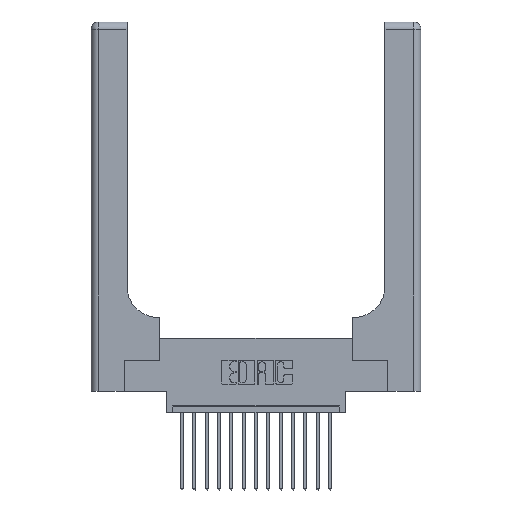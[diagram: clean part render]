
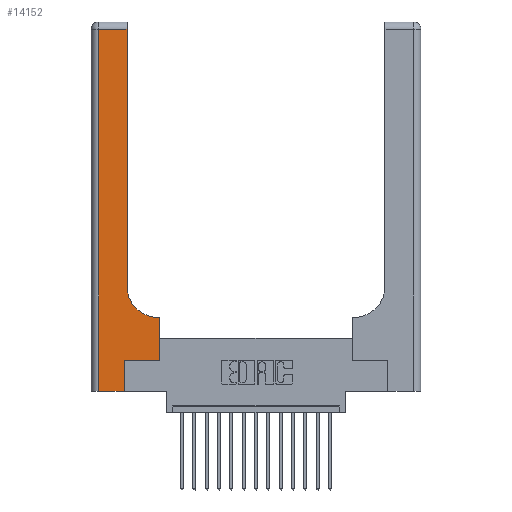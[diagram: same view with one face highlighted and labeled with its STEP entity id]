
A CAD part, top view. The second image highlights one B-rep face of the part: STEP entity #14152.
In plain terms, the highlighted planar face has unit normal (0, 0, 1).
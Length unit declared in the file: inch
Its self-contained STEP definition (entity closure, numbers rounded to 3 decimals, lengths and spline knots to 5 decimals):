
#20 = LINE ( 'NONE', #16903, #18174 ) ;
#531 = EDGE_CURVE ( 'NONE', #2911, #3410, #15299, .T. ) ;
#807 = DIRECTION ( 'NONE',  ( -1., 0., 0. ) ) ;
#1036 = EDGE_CURVE ( 'NONE', #12377, #18561, #9142, .T. ) ;
#1433 = ORIENTED_EDGE ( 'NONE', *, *, #1036, .T. ) ;
#1596 = DIRECTION ( 'NONE',  ( 1., 0., 0. ) ) ;
#1735 = VECTOR ( 'NONE', #10958, 39.37008 ) ;
#1915 = VERTEX_POINT ( 'NONE', #6705 ) ;
#2911 = VERTEX_POINT ( 'NONE', #12898 ) ;
#3210 = FACE_OUTER_BOUND ( 'NONE', #6744, .T. ) ;
#3400 = CARTESIAN_POINT ( 'NONE',  ( 0.5415, 0.85, 0.37 ) ) ;
#3410 = VERTEX_POINT ( 'NONE', #11936 ) ;
#3576 = DIRECTION ( 'NONE',  ( 0., 1., 0. ) ) ;
#4557 = EDGE_CURVE ( 'NONE', #17406, #17533, #11601, .T. ) ;
#5170 = CARTESIAN_POINT ( 'NONE',  ( 0.5585, 0.25, 0.37 ) ) ;
#5203 = ORIENTED_EDGE ( 'NONE', *, *, #15458, .T. ) ;
#5478 = ORIENTED_EDGE ( 'NONE', *, *, #6938, .T. ) ;
#5846 = ORIENTED_EDGE ( 'NONE', *, *, #531, .T. ) ;
#6306 = VECTOR ( 'NONE', #13634, 39.37008 ) ;
#6356 = LINE ( 'NONE', #17411, #8203 ) ;
#6435 = AXIS2_PLACEMENT_3D ( 'NONE', #12868, #6892, #14323 ) ;
#6705 = CARTESIAN_POINT ( 'NONE',  ( 0.269, 0.25, 0.37 ) ) ;
#6744 = EDGE_LOOP ( 'NONE', ( #8381, #10017, #5203, #9427, #14800, #14007, #1433, #5478, #5846 ) ) ;
#6892 = DIRECTION ( 'NONE',  ( 0., 0., -1. ) ) ;
#6938 = EDGE_CURVE ( 'NONE', #18561, #2911, #20, .T. ) ;
#7026 = PLANE ( 'NONE',  #6435 ) ;
#7500 = CARTESIAN_POINT ( 'NONE',  ( 0., 0., 0.37 ) ) ;
#7630 = DIRECTION ( 'NONE',  ( 1., 0., 0. ) ) ;
#7783 = CARTESIAN_POINT ( 'NONE',  ( 0.269, 0.25, 0.37 ) ) ;
#7818 = DIRECTION ( 'NONE',  ( 0., 0., -1. ) ) ;
#8203 = VECTOR ( 'NONE', #11316, 39.37008 ) ;
#8381 = ORIENTED_EDGE ( 'NONE', *, *, #13982, .T. ) ;
#8624 = EDGE_CURVE ( 'NONE', #17237, #17893, #17671, .T. ) ;
#9088 = CARTESIAN_POINT ( 'NONE',  ( 0.269, 0., 0.37 ) ) ;
#9142 = LINE ( 'NONE', #9435, #13070 ) ;
#9427 = ORIENTED_EDGE ( 'NONE', *, *, #4557, .T. ) ;
#9435 = CARTESIAN_POINT ( 'NONE',  ( 0.5585, 0.25, 0.37 ) ) ;
#9648 = EDGE_CURVE ( 'NONE', #17533, #1915, #11663, .T. ) ;
#10017 = ORIENTED_EDGE ( 'NONE', *, *, #8624, .T. ) ;
#10144 = CARTESIAN_POINT ( 'NONE',  ( 0.2915, 2.94, 0.37 ) ) ;
#10468 = DIRECTION ( 'NONE',  ( 0., 1., 0. ) ) ;
#10664 = VECTOR ( 'NONE', #1596, 39.37008 ) ;
#10958 = DIRECTION ( 'NONE',  ( 0., 1., 0. ) ) ;
#11316 = DIRECTION ( 'NONE',  ( 0., -1., 0. ) ) ;
#11601 = LINE ( 'NONE', #7500, #10664 ) ;
#11663 = LINE ( 'NONE', #9088, #13721 ) ;
#11936 = CARTESIAN_POINT ( 'NONE',  ( 0.2915, 0.85, 0.37 ) ) ;
#12377 = VERTEX_POINT ( 'NONE', #5170 ) ;
#12868 = CARTESIAN_POINT ( 'NONE',  ( 0., 3., 0.37 ) ) ;
#12898 = CARTESIAN_POINT ( 'NONE',  ( 0.5415, 0.6, 0.37 ) ) ;
#13070 = VECTOR ( 'NONE', #3576, 39.37008 ) ;
#13163 = AXIS2_PLACEMENT_3D ( 'NONE', #3400, #7818, #7630 ) ;
#13435 = CARTESIAN_POINT ( 'NONE',  ( 0.06, 0., 0.37 ) ) ;
#13634 = DIRECTION ( 'NONE',  ( 1., 0., 0. ) ) ;
#13721 = VECTOR ( 'NONE', #10468, 39.37008 ) ;
#13982 = EDGE_CURVE ( 'NONE', #3410, #17237, #17121, .T. ) ;
#14007 = ORIENTED_EDGE ( 'NONE', *, *, #16879, .T. ) ;
#14077 = CARTESIAN_POINT ( 'NONE',  ( 0.2915, 3., 0.37 ) ) ;
#14152 = ADVANCED_FACE ( 'NONE', ( #3210 ), #7026, .F. ) ;
#14323 = DIRECTION ( 'NONE',  ( -1., 0., 0. ) ) ;
#14800 = ORIENTED_EDGE ( 'NONE', *, *, #9648, .T. ) ;
#15299 = CIRCLE ( 'NONE', #13163, 0.25 ) ;
#15458 = EDGE_CURVE ( 'NONE', #17893, #17406, #6356, .T. ) ;
#15714 = CARTESIAN_POINT ( 'NONE',  ( 0.06, 2.94, 0.37 ) ) ;
#16423 = DIRECTION ( 'NONE',  ( -1., 0., 0. ) ) ;
#16533 = VECTOR ( 'NONE', #16423, 39.37008 ) ;
#16641 = CARTESIAN_POINT ( 'NONE',  ( 0.269, 0., 0.37 ) ) ;
#16879 = EDGE_CURVE ( 'NONE', #1915, #12377, #18745, .T. ) ;
#16903 = CARTESIAN_POINT ( 'NONE',  ( 0.2915, 0.6, 0.37 ) ) ;
#17121 = LINE ( 'NONE', #14077, #1735 ) ;
#17237 = VERTEX_POINT ( 'NONE', #10144 ) ;
#17406 = VERTEX_POINT ( 'NONE', #13435 ) ;
#17411 = CARTESIAN_POINT ( 'NONE',  ( 0.06, 3., 0.37 ) ) ;
#17533 = VERTEX_POINT ( 'NONE', #16641 ) ;
#17671 = LINE ( 'NONE', #17788, #16533 ) ;
#17788 = CARTESIAN_POINT ( 'NONE',  ( 0., 2.94, 0.37 ) ) ;
#17893 = VERTEX_POINT ( 'NONE', #15714 ) ;
#18174 = VECTOR ( 'NONE', #807, 39.37008 ) ;
#18561 = VERTEX_POINT ( 'NONE', #18823 ) ;
#18745 = LINE ( 'NONE', #7783, #6306 ) ;
#18823 = CARTESIAN_POINT ( 'NONE',  ( 0.5585, 0.6, 0.37 ) ) ;
